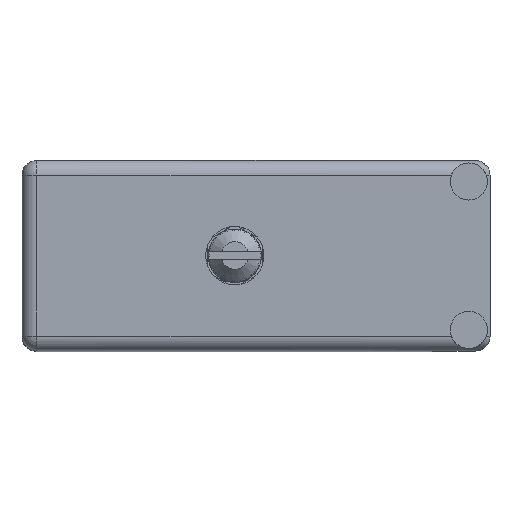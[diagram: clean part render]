
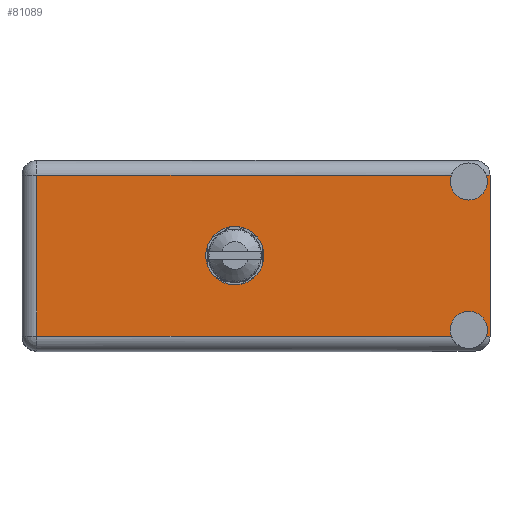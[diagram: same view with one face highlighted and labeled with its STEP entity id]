
A CAD part, top view. The second image highlights one B-rep face of the part: STEP entity #81089.
In plain terms, the highlighted face is planar.
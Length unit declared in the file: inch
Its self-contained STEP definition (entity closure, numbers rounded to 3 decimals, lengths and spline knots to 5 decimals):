
#788 = VECTOR ( 'NONE', #48877, 39.37008 ) ;
#1272 = FACE_OUTER_BOUND ( 'NONE', #85603, .T. ) ;
#1296 = ORIENTED_EDGE ( 'NONE', *, *, #16666, .T. ) ;
#2463 = LINE ( 'NONE', #4498, #25278 ) ;
#2934 = CARTESIAN_POINT ( 'NONE',  ( 1.104, 1.466, 0.35 ) ) ;
#3071 = CARTESIAN_POINT ( 'NONE',  ( -0.934, 1.466, -0.4495 ) ) ;
#3982 = DIRECTION ( 'NONE',  ( 0., 0., 1. ) ) ;
#4366 = LINE ( 'NONE', #63707, #78215 ) ;
#4498 = CARTESIAN_POINT ( 'NONE',  ( 1.204, 1.466, 0.3795 ) ) ;
#6879 = ORIENTED_EDGE ( 'NONE', *, *, #91251, .T. ) ;
#8483 = VERTEX_POINT ( 'NONE', #72646 ) ;
#9508 = EDGE_CURVE ( 'NONE', #24663, #90307, #77812, .T. ) ;
#10738 = DIRECTION ( 'NONE',  ( 0., 1., 0. ) ) ;
#13931 = CIRCLE ( 'NONE', #69974, 0.1375 ) ;
#15037 = CARTESIAN_POINT ( 'NONE',  ( 1.104, 1.466, 0.35 ) ) ;
#15454 = DIRECTION ( 'NONE',  ( 0., 1., 0. ) ) ;
#16666 = EDGE_CURVE ( 'NONE', #95955, #85630, #64338, .T. ) ;
#16961 = AXIS2_PLACEMENT_3D ( 'NONE', #105247, #15454, #56712 ) ;
#18393 = EDGE_CURVE ( 'NONE', #95955, #90307, #27164, .T. ) ;
#18433 = VECTOR ( 'NONE', #101011, 39.37008 ) ;
#20269 = ORIENTED_EDGE ( 'NONE', *, *, #48785, .F. ) ;
#21033 = CARTESIAN_POINT ( 'NONE',  ( -0.934, 1.466, 0.3795 ) ) ;
#21553 = DIRECTION ( 'NONE',  ( 0., 1., 0. ) ) ;
#22587 = CIRCLE ( 'NONE', #98281, 0.0875 ) ;
#24195 = ORIENTED_EDGE ( 'NONE', *, *, #96951, .T. ) ;
#24663 = VERTEX_POINT ( 'NONE', #81347 ) ;
#25278 = VECTOR ( 'NONE', #37504, 39.37008 ) ;
#27164 = LINE ( 'NONE', #100011, #97343 ) ;
#27523 = DIRECTION ( 'NONE',  ( 0., 1., 0. ) ) ;
#27936 = EDGE_CURVE ( 'NONE', #83865, #39070, #45179, .T. ) ;
#28207 = AXIS2_PLACEMENT_3D ( 'NONE', #101550, #29171, #68677 ) ;
#28225 = EDGE_CURVE ( 'NONE', #24663, #96876, #77030, .T. ) ;
#28666 = CARTESIAN_POINT ( 'NONE',  ( 0., 1.466, 0. ) ) ;
#29171 = DIRECTION ( 'NONE',  ( 0., 1., 0. ) ) ;
#29459 = ORIENTED_EDGE ( 'NONE', *, *, #49854, .F. ) ;
#33562 = VERTEX_POINT ( 'NONE', #85824 ) ;
#35008 = ORIENTED_EDGE ( 'NONE', *, *, #46432, .F. ) ;
#35159 = CARTESIAN_POINT ( 'NONE',  ( 1.02162, 1.466, 0.3795 ) ) ;
#37504 = DIRECTION ( 'NONE',  ( 1., 0., 0. ) ) ;
#37685 = CARTESIAN_POINT ( 'NONE',  ( 0., 1.466, 0. ) ) ;
#39070 = VERTEX_POINT ( 'NONE', #21033 ) ;
#39210 = CARTESIAN_POINT ( 'NONE',  ( 1.18638, 1.466, -0.3795 ) ) ;
#44351 = ORIENTED_EDGE ( 'NONE', *, *, #27936, .T. ) ;
#44487 = DIRECTION ( 'NONE',  ( 1., 0., 0. ) ) ;
#44784 = CARTESIAN_POINT ( 'NONE',  ( 1.204, 1.466, 0.3795 ) ) ;
#45128 = PLANE ( 'NONE',  #28207 ) ;
#45179 = LINE ( 'NONE', #3071, #18433 ) ;
#46432 = EDGE_CURVE ( 'NONE', #92530, #33562, #13931, .T. ) ;
#47905 = VERTEX_POINT ( 'NONE', #35159 ) ;
#48785 = EDGE_CURVE ( 'NONE', #72104, #85630, #22587, .T. ) ;
#48877 = DIRECTION ( 'NONE',  ( -1., 0., 0. ) ) ;
#49854 = EDGE_CURVE ( 'NONE', #96876, #47905, #66972, .T. ) ;
#51991 = CARTESIAN_POINT ( 'NONE',  ( 1.204, 1.466, 0.3795 ) ) ;
#56551 = EDGE_CURVE ( 'NONE', #33562, #92530, #73678, .T. ) ;
#56712 = DIRECTION ( 'NONE',  ( 0., 0., 1. ) ) ;
#57316 = AXIS2_PLACEMENT_3D ( 'NONE', #15037, #79489, #104162 ) ;
#63707 = CARTESIAN_POINT ( 'NONE',  ( -1.004, 1.466, -0.3795 ) ) ;
#64338 = LINE ( 'NONE', #89900, #788 ) ;
#64987 = AXIS2_PLACEMENT_3D ( 'NONE', #28666, #21553, #102448 ) ;
#66972 = CIRCLE ( 'NONE', #57316, 0.0875 ) ;
#67228 = CARTESIAN_POINT ( 'NONE',  ( -0.934, 1.466, -0.3795 ) ) ;
#67380 = FACE_BOUND ( 'NONE', #88657, .T. ) ;
#68677 = DIRECTION ( 'NONE',  ( -1., 0., 0. ) ) ;
#69626 = CARTESIAN_POINT ( 'NONE',  ( 1.204, 1.466, -0.3795 ) ) ;
#69934 = ORIENTED_EDGE ( 'NONE', *, *, #9508, .T. ) ;
#69974 = AXIS2_PLACEMENT_3D ( 'NONE', #37685, #85817, #3982 ) ;
#71354 = ORIENTED_EDGE ( 'NONE', *, *, #90947, .F. ) ;
#72104 = VERTEX_POINT ( 'NONE', #101253 ) ;
#72646 = CARTESIAN_POINT ( 'NONE',  ( 1.02162, 1.466, -0.3795 ) ) ;
#73678 = CIRCLE ( 'NONE', #64987, 0.1375 ) ;
#74210 = ORIENTED_EDGE ( 'NONE', *, *, #56551, .F. ) ;
#76073 = CARTESIAN_POINT ( 'NONE',  ( 1.104, 1.466, 0.2625 ) ) ;
#76340 = CARTESIAN_POINT ( 'NONE',  ( 1.104, 1.466, -0.35 ) ) ;
#76969 = CIRCLE ( 'NONE', #16961, 0.0875 ) ;
#77030 = CIRCLE ( 'NONE', #92262, 0.0875 ) ;
#77812 = LINE ( 'NONE', #51991, #102085 ) ;
#78215 = VECTOR ( 'NONE', #104766, 39.37008 ) ;
#79489 = DIRECTION ( 'NONE',  ( 0., 1., 0. ) ) ;
#81089 = ADVANCED_FACE ( 'NONE', ( #67380, #1272 ), #45128, .T. ) ;
#81347 = CARTESIAN_POINT ( 'NONE',  ( 1.18638, 1.466, 0.3795 ) ) ;
#83000 = DIRECTION ( 'NONE',  ( 0., 0., 1. ) ) ;
#83865 = VERTEX_POINT ( 'NONE', #67228 ) ;
#84040 = ORIENTED_EDGE ( 'NONE', *, *, #28225, .F. ) ;
#84495 = DIRECTION ( 'NONE',  ( 0., 0., 1. ) ) ;
#85603 = EDGE_LOOP ( 'NONE', ( #24195, #29459, #84040, #69934, #88009, #1296, #20269, #71354, #6879, #44351 ) ) ;
#85630 = VERTEX_POINT ( 'NONE', #39210 ) ;
#85817 = DIRECTION ( 'NONE',  ( 0., 1., 0. ) ) ;
#85824 = CARTESIAN_POINT ( 'NONE',  ( 0., 1.466, -0.1375 ) ) ;
#88009 = ORIENTED_EDGE ( 'NONE', *, *, #18393, .F. ) ;
#88657 = EDGE_LOOP ( 'NONE', ( #35008, #74210 ) ) ;
#89900 = CARTESIAN_POINT ( 'NONE',  ( -1.004, 1.466, -0.3795 ) ) ;
#90307 = VERTEX_POINT ( 'NONE', #44784 ) ;
#90947 = EDGE_CURVE ( 'NONE', #8483, #72104, #76969, .T. ) ;
#91251 = EDGE_CURVE ( 'NONE', #8483, #83865, #4366, .T. ) ;
#92262 = AXIS2_PLACEMENT_3D ( 'NONE', #2934, #10738, #83000 ) ;
#92530 = VERTEX_POINT ( 'NONE', #101949 ) ;
#95955 = VERTEX_POINT ( 'NONE', #69626 ) ;
#96876 = VERTEX_POINT ( 'NONE', #76073 ) ;
#96951 = EDGE_CURVE ( 'NONE', #39070, #47905, #2463, .T. ) ;
#97343 = VECTOR ( 'NONE', #98590, 39.37008 ) ;
#98281 = AXIS2_PLACEMENT_3D ( 'NONE', #76340, #27523, #84495 ) ;
#98590 = DIRECTION ( 'NONE',  ( 0., 0., 1. ) ) ;
#100011 = CARTESIAN_POINT ( 'NONE',  ( 1.204, 1.466, 0.4495 ) ) ;
#101011 = DIRECTION ( 'NONE',  ( 0., 0., 1. ) ) ;
#101253 = CARTESIAN_POINT ( 'NONE',  ( 1.104, 1.466, -0.2625 ) ) ;
#101550 = CARTESIAN_POINT ( 'NONE',  ( -1.004, 1.466, -0.4495 ) ) ;
#101949 = CARTESIAN_POINT ( 'NONE',  ( 0., 1.466, 0.1375 ) ) ;
#102085 = VECTOR ( 'NONE', #44487, 39.37008 ) ;
#102448 = DIRECTION ( 'NONE',  ( 0., 0., 1. ) ) ;
#104162 = DIRECTION ( 'NONE',  ( 0., 0., 1. ) ) ;
#104766 = DIRECTION ( 'NONE',  ( -1., 0., 0. ) ) ;
#105247 = CARTESIAN_POINT ( 'NONE',  ( 1.104, 1.466, -0.35 ) ) ;
